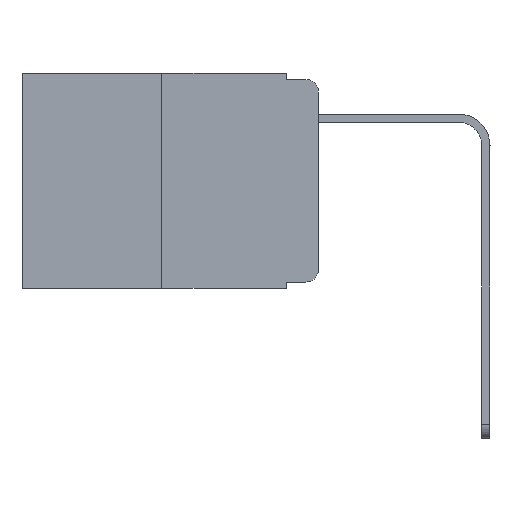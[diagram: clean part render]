
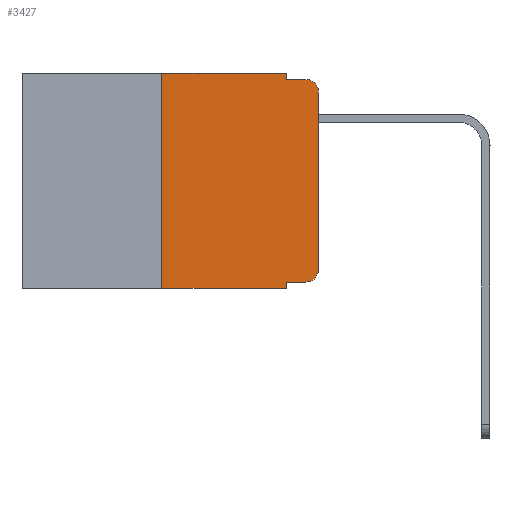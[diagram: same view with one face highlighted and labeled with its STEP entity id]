
A CAD part, left-side view. The second image highlights one B-rep face of the part: STEP entity #3427.
In plain terms, the highlighted planar face has unit normal (-1, 0, 0).
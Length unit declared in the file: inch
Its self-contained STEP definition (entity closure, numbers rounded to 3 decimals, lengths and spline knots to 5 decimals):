
#271 = ORIENTED_EDGE ( 'NONE', *, *, #12688, .T. ) ;
#275 = VERTEX_POINT ( 'NONE', #906 ) ;
#752 = EDGE_CURVE ( 'NONE', #16978, #2656, #17105, .T. ) ;
#906 = CARTESIAN_POINT ( 'NONE',  ( 0., 0.02, -0.01 ) ) ;
#947 = CARTESIAN_POINT ( 'NONE',  ( 0., 0.051, 0. ) ) ;
#1100 = EDGE_LOOP ( 'NONE', ( #8472, #271, #15128, #11858, #5664, #11843, #3123, #3063, #16916, #9842 ) ) ;
#1170 = CARTESIAN_POINT ( 'NONE',  ( 0., 0.473, -0.343 ) ) ;
#1269 = VERTEX_POINT ( 'NONE', #947 ) ;
#1469 = CARTESIAN_POINT ( 'NONE',  ( 0., 0.473, 0. ) ) ;
#1921 = CARTESIAN_POINT ( 'NONE',  ( 0., 0.051, -0.01 ) ) ;
#1992 = EDGE_CURVE ( 'NONE', #1269, #8454, #12245, .T. ) ;
#2050 = DIRECTION ( 'NONE',  ( 0., -1., 0. ) ) ;
#2175 = EDGE_CURVE ( 'NONE', #13940, #1269, #7678, .T. ) ;
#2640 = VECTOR ( 'NONE', #19622, 39.37008 ) ;
#2656 = VERTEX_POINT ( 'NONE', #5572 ) ;
#2729 = LINE ( 'NONE', #17305, #8980 ) ;
#2761 = VECTOR ( 'NONE', #18172, 39.37008 ) ;
#2924 = CARTESIAN_POINT ( 'NONE',  ( 0., 0.02, -0.03 ) ) ;
#2928 = CIRCLE ( 'NONE', #7010, 0.02 ) ;
#3063 = ORIENTED_EDGE ( 'NONE', *, *, #8991, .F. ) ;
#3115 = DIRECTION ( 'NONE',  ( -1., 0., 0. ) ) ;
#3123 = ORIENTED_EDGE ( 'NONE', *, *, #752, .T. ) ;
#3217 = PLANE ( 'NONE',  #10138 ) ;
#3427 = ADVANCED_FACE ( 'NONE', ( #12190 ), #3217, .F. ) ;
#3472 = CARTESIAN_POINT ( 'NONE',  ( 0., 0.02, -0.333 ) ) ;
#3834 = LINE ( 'NONE', #11984, #11753 ) ;
#3979 = EDGE_CURVE ( 'NONE', #19871, #5969, #13630, .T. ) ;
#4552 = DIRECTION ( 'NONE',  ( 0., 0., -1. ) ) ;
#4882 = DIRECTION ( 'NONE',  ( 0., 0., -1. ) ) ;
#5436 = VECTOR ( 'NONE', #10709, 39.37008 ) ;
#5506 = CARTESIAN_POINT ( 'NONE',  ( 0., 0.25, -0.343 ) ) ;
#5572 = CARTESIAN_POINT ( 'NONE',  ( 0., 0.051, -0.343 ) ) ;
#5609 = VERTEX_POINT ( 'NONE', #10579 ) ;
#5664 = ORIENTED_EDGE ( 'NONE', *, *, #2175, .F. ) ;
#5969 = VERTEX_POINT ( 'NONE', #3472 ) ;
#6600 = DIRECTION ( 'NONE',  ( 0., 0., -1. ) ) ;
#7010 = AXIS2_PLACEMENT_3D ( 'NONE', #2924, #3115, #4552 ) ;
#7238 = EDGE_CURVE ( 'NONE', #8454, #275, #15533, .T. ) ;
#7546 = CARTESIAN_POINT ( 'NONE',  ( 0., 0.051, -0.01 ) ) ;
#7678 = LINE ( 'NONE', #18981, #15359 ) ;
#7852 = EDGE_CURVE ( 'NONE', #16978, #13940, #10938, .T. ) ;
#8454 = VERTEX_POINT ( 'NONE', #7546 ) ;
#8472 = ORIENTED_EDGE ( 'NONE', *, *, #16483, .T. ) ;
#8980 = VECTOR ( 'NONE', #4882, 39.37008 ) ;
#8991 = EDGE_CURVE ( 'NONE', #19871, #2656, #2729, .T. ) ;
#9215 = CARTESIAN_POINT ( 'NONE',  ( 0., 0.051, -0.333 ) ) ;
#9272 = DIRECTION ( 'NONE',  ( 0., 0., -1. ) ) ;
#9842 = ORIENTED_EDGE ( 'NONE', *, *, #12598, .T. ) ;
#10138 = AXIS2_PLACEMENT_3D ( 'NONE', #1469, #10767, #9272 ) ;
#10406 = DIRECTION ( 'NONE',  ( 0., -1., 0. ) ) ;
#10579 = CARTESIAN_POINT ( 'NONE',  ( 0., 0., -0.03 ) ) ;
#10709 = DIRECTION ( 'NONE',  ( 0., -1., 0. ) ) ;
#10767 = DIRECTION ( 'NONE',  ( 1., 0., 0. ) ) ;
#10938 = LINE ( 'NONE', #18107, #2761 ) ;
#11753 = VECTOR ( 'NONE', #12240, 39.37008 ) ;
#11805 = CARTESIAN_POINT ( 'NONE',  ( 0., 0.051, 0. ) ) ;
#11843 = ORIENTED_EDGE ( 'NONE', *, *, #7852, .F. ) ;
#11858 = ORIENTED_EDGE ( 'NONE', *, *, #1992, .F. ) ;
#11984 = CARTESIAN_POINT ( 'NONE',  ( 0., 0., 0. ) ) ;
#12190 = FACE_OUTER_BOUND ( 'NONE', #1100, .T. ) ;
#12240 = DIRECTION ( 'NONE',  ( 0., 0., 1. ) ) ;
#12245 = LINE ( 'NONE', #11805, #2640 ) ;
#12598 = EDGE_CURVE ( 'NONE', #5969, #12875, #14944, .T. ) ;
#12688 = EDGE_CURVE ( 'NONE', #5609, #275, #2928, .T. ) ;
#12875 = VERTEX_POINT ( 'NONE', #13894 ) ;
#13630 = LINE ( 'NONE', #9215, #5436 ) ;
#13894 = CARTESIAN_POINT ( 'NONE',  ( 0., 0., -0.313 ) ) ;
#13940 = VERTEX_POINT ( 'NONE', #18697 ) ;
#14382 = DIRECTION ( 'NONE',  ( 0., -1., 0. ) ) ;
#14944 = CIRCLE ( 'NONE', #19400, 0.02 ) ;
#15128 = ORIENTED_EDGE ( 'NONE', *, *, #7238, .F. ) ;
#15359 = VECTOR ( 'NONE', #14382, 39.37008 ) ;
#15533 = LINE ( 'NONE', #1921, #18912 ) ;
#15795 = DIRECTION ( 'NONE',  ( -1., 0., 0. ) ) ;
#16483 = EDGE_CURVE ( 'NONE', #12875, #5609, #3834, .T. ) ;
#16916 = ORIENTED_EDGE ( 'NONE', *, *, #3979, .T. ) ;
#16978 = VERTEX_POINT ( 'NONE', #5506 ) ;
#17105 = LINE ( 'NONE', #1170, #19060 ) ;
#17278 = CARTESIAN_POINT ( 'NONE',  ( 0., 0.051, -0.333 ) ) ;
#17305 = CARTESIAN_POINT ( 'NONE',  ( 0., 0.051, 0. ) ) ;
#17337 = CARTESIAN_POINT ( 'NONE',  ( 0., 0.02, -0.313 ) ) ;
#18107 = CARTESIAN_POINT ( 'NONE',  ( 0., 0.25, 0. ) ) ;
#18172 = DIRECTION ( 'NONE',  ( 0., 0., 1. ) ) ;
#18697 = CARTESIAN_POINT ( 'NONE',  ( 0., 0.25, 0. ) ) ;
#18912 = VECTOR ( 'NONE', #2050, 39.37008 ) ;
#18981 = CARTESIAN_POINT ( 'NONE',  ( 0., 0.473, 0. ) ) ;
#19060 = VECTOR ( 'NONE', #10406, 39.37008 ) ;
#19400 = AXIS2_PLACEMENT_3D ( 'NONE', #17337, #15795, #6600 ) ;
#19622 = DIRECTION ( 'NONE',  ( 0., 0., -1. ) ) ;
#19871 = VERTEX_POINT ( 'NONE', #17278 ) ;
